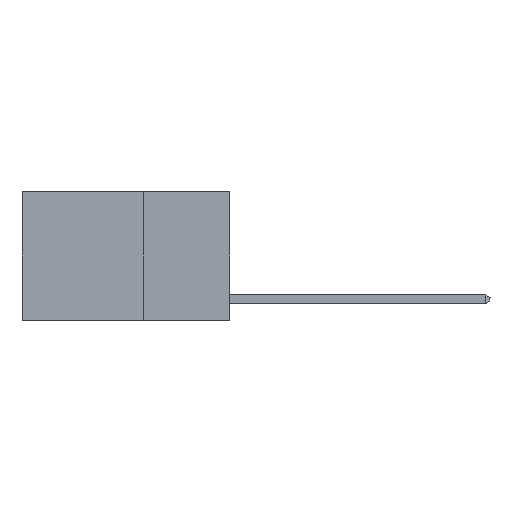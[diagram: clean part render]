
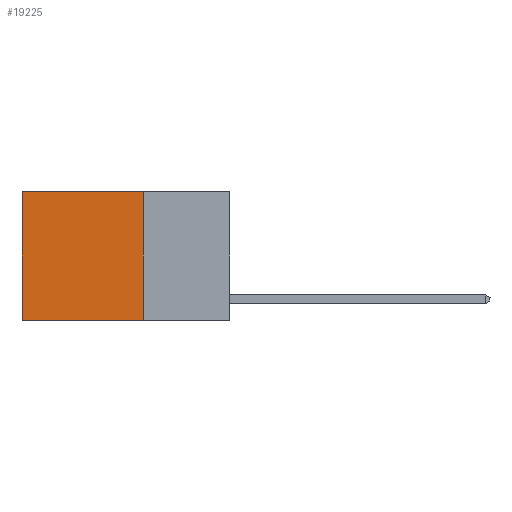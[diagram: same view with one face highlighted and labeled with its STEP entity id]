
A CAD part, left-side view. The second image highlights one B-rep face of the part: STEP entity #19225.
In plain terms, the highlighted planar face has unit normal (-1, 0, 0).
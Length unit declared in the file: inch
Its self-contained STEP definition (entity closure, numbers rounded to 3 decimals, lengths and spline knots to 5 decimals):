
#1489 = VECTOR ( 'NONE', #11217, 39.37008 ) ;
#1977 = LINE ( 'NONE', #17830, #1489 ) ;
#2149 = DIRECTION ( 'NONE',  ( 1., 0., 0. ) ) ;
#3044 = CARTESIAN_POINT ( 'NONE',  ( 0.2625, 0.25, 0. ) ) ;
#4183 = CARTESIAN_POINT ( 'NONE',  ( 0.2625, 0.6, 0. ) ) ;
#6733 = VERTEX_POINT ( 'NONE', #19867 ) ;
#7461 = FACE_OUTER_BOUND ( 'NONE', #13331, .T. ) ;
#8197 = ORIENTED_EDGE ( 'NONE', *, *, #20668, .F. ) ;
#8623 = LINE ( 'NONE', #17149, #12336 ) ;
#9844 = DIRECTION ( 'NONE',  ( 0., 1., 0. ) ) ;
#11217 = DIRECTION ( 'NONE',  ( 0., 0., -1. ) ) ;
#12047 = CARTESIAN_POINT ( 'NONE',  ( 0.2625, 0.25, 0. ) ) ;
#12336 = VECTOR ( 'NONE', #17004, 39.37008 ) ;
#12527 = VERTEX_POINT ( 'NONE', #21710 ) ;
#13035 = CARTESIAN_POINT ( 'NONE',  ( 0.2625, 0.25, -0.37 ) ) ;
#13111 = DIRECTION ( 'NONE',  ( 0., 0., -1. ) ) ;
#13135 = DIRECTION ( 'NONE',  ( 0., 0., -1. ) ) ;
#13331 = EDGE_LOOP ( 'NONE', ( #16745, #8197, #26102, #22275 ) ) ;
#14403 = VECTOR ( 'NONE', #9844, 39.37008 ) ;
#15354 = CARTESIAN_POINT ( 'NONE',  ( 0.2625, 0.25, 0. ) ) ;
#15374 = VERTEX_POINT ( 'NONE', #13035 ) ;
#15601 = AXIS2_PLACEMENT_3D ( 'NONE', #15354, #2149, #13135 ) ;
#16268 = EDGE_CURVE ( 'NONE', #26280, #15374, #1977, .T. ) ;
#16292 = EDGE_CURVE ( 'NONE', #6733, #12527, #24251, .T. ) ;
#16745 = ORIENTED_EDGE ( 'NONE', *, *, #16292, .T. ) ;
#16761 = LINE ( 'NONE', #12047, #14403 ) ;
#17004 = DIRECTION ( 'NONE',  ( 0., 1., 0. ) ) ;
#17149 = CARTESIAN_POINT ( 'NONE',  ( 0.2625, 0.25, -0.37 ) ) ;
#17830 = CARTESIAN_POINT ( 'NONE',  ( 0.2625, 0.25, 0. ) ) ;
#19225 = ADVANCED_FACE ( 'NONE', ( #7461 ), #19752, .F. ) ;
#19752 = PLANE ( 'NONE',  #15601 ) ;
#19867 = CARTESIAN_POINT ( 'NONE',  ( 0.2625, 0.6, 0. ) ) ;
#20668 = EDGE_CURVE ( 'NONE', #15374, #12527, #8623, .T. ) ;
#21710 = CARTESIAN_POINT ( 'NONE',  ( 0.2625, 0.6, -0.37 ) ) ;
#22275 = ORIENTED_EDGE ( 'NONE', *, *, #26115, .T. ) ;
#24251 = LINE ( 'NONE', #4183, #24888 ) ;
#24888 = VECTOR ( 'NONE', #13111, 39.37008 ) ;
#26102 = ORIENTED_EDGE ( 'NONE', *, *, #16268, .F. ) ;
#26115 = EDGE_CURVE ( 'NONE', #26280, #6733, #16761, .T. ) ;
#26280 = VERTEX_POINT ( 'NONE', #3044 ) ;
